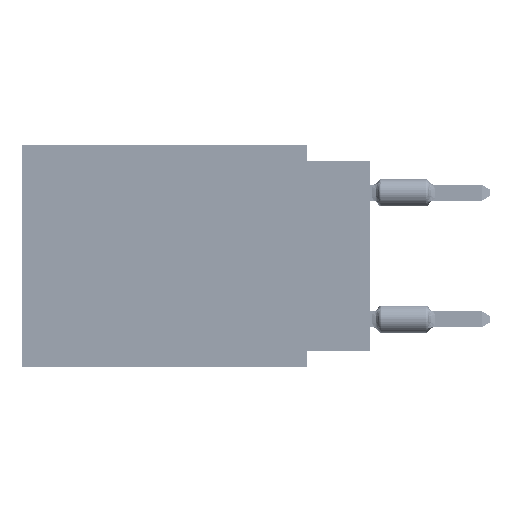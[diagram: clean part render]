
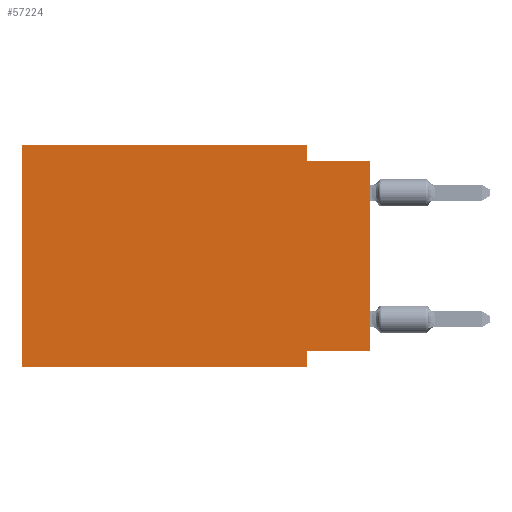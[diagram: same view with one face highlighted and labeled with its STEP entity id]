
A CAD part, left-side view. The second image highlights one B-rep face of the part: STEP entity #57224.
In plain terms, the highlighted planar face has unit normal (-1, 0, 0).
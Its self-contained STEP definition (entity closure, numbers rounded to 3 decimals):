
#6 = CARTESIAN_POINT ( 'NONE',  ( 0., 0., -8.255 ) ) ;
#1373 = CARTESIAN_POINT ( 'NONE',  ( 0., 13.97, -8.89 ) ) ;
#1669 = DIRECTION ( 'NONE',  ( 0., -1., 0. ) ) ;
#2121 = CARTESIAN_POINT ( 'NONE',  ( 0., 13.97, 0. ) ) ;
#2749 = VECTOR ( 'NONE', #61164, 1000. ) ;
#2925 = VERTEX_POINT ( 'NONE', #60338 ) ;
#3912 = VECTOR ( 'NONE', #45170, 1000. ) ;
#4135 = VERTEX_POINT ( 'NONE', #33425 ) ;
#4671 = ORIENTED_EDGE ( 'NONE', *, *, #45342, .F. ) ;
#5426 = VECTOR ( 'NONE', #49405, 1000. ) ;
#6411 = VECTOR ( 'NONE', #42170, 1000. ) ;
#7869 = VERTEX_POINT ( 'NONE', #43245 ) ;
#8505 = VECTOR ( 'NONE', #1669, 1000. ) ;
#12434 = EDGE_LOOP ( 'NONE', ( #36051, #48509, #4671, #23548, #65354, #19187, #33474, #23314 ) ) ;
#13574 = DIRECTION ( 'NONE',  ( 1., 0., 0. ) ) ;
#13712 = LINE ( 'NONE', #67675, #30458 ) ;
#14795 = VERTEX_POINT ( 'NONE', #1373 ) ;
#16753 = VERTEX_POINT ( 'NONE', #24791 ) ;
#18209 = PLANE ( 'NONE',  #68931 ) ;
#19187 = ORIENTED_EDGE ( 'NONE', *, *, #57685, .T. ) ;
#23314 = ORIENTED_EDGE ( 'NONE', *, *, #55597, .F. ) ;
#23548 = ORIENTED_EDGE ( 'NONE', *, *, #30629, .F. ) ;
#23978 = LINE ( 'NONE', #46835, #34636 ) ;
#24791 = CARTESIAN_POINT ( 'NONE',  ( 0., 2.54, -8.255 ) ) ;
#28027 = DIRECTION ( 'NONE',  ( 0., -1., 0. ) ) ;
#29636 = FACE_OUTER_BOUND ( 'NONE', #12434, .T. ) ;
#30458 = VECTOR ( 'NONE', #46916, 1000. ) ;
#30629 = EDGE_CURVE ( 'NONE', #2925, #41798, #59669, .T. ) ;
#33425 = CARTESIAN_POINT ( 'NONE',  ( 0., 2.54, -8.89 ) ) ;
#33474 = ORIENTED_EDGE ( 'NONE', *, *, #55170, .F. ) ;
#34028 = CARTESIAN_POINT ( 'NONE',  ( 0., 0., 0. ) ) ;
#34437 = LINE ( 'NONE', #40511, #3912 ) ;
#34636 = VECTOR ( 'NONE', #28027, 1000. ) ;
#36051 = ORIENTED_EDGE ( 'NONE', *, *, #60522, .T. ) ;
#38106 = VECTOR ( 'NONE', #42697, 1000. ) ;
#38647 = LINE ( 'NONE', #39332, #2749 ) ;
#39332 = CARTESIAN_POINT ( 'NONE',  ( 0., 0., -8.255 ) ) ;
#40489 = CARTESIAN_POINT ( 'NONE',  ( 0., 2.54, -0.635 ) ) ;
#40511 = CARTESIAN_POINT ( 'NONE',  ( 0., 13.97, 0. ) ) ;
#41798 = VERTEX_POINT ( 'NONE', #46717 ) ;
#42170 = DIRECTION ( 'NONE',  ( 0., -1., 0. ) ) ;
#42697 = DIRECTION ( 'NONE',  ( 0., 0., -1. ) ) ;
#43245 = CARTESIAN_POINT ( 'NONE',  ( 0., 0., -0.635 ) ) ;
#45170 = DIRECTION ( 'NONE',  ( 0., 0., 1. ) ) ;
#45342 = EDGE_CURVE ( 'NONE', #41798, #52686, #13712, .T. ) ;
#46717 = CARTESIAN_POINT ( 'NONE',  ( 0., 2.54, 0. ) ) ;
#46835 = CARTESIAN_POINT ( 'NONE',  ( 0., 0., -0.635 ) ) ;
#46916 = DIRECTION ( 'NONE',  ( 0., 0., -1. ) ) ;
#48509 = ORIENTED_EDGE ( 'NONE', *, *, #54257, .F. ) ;
#49405 = DIRECTION ( 'NONE',  ( 0., 0., 1. ) ) ;
#50657 = CARTESIAN_POINT ( 'NONE',  ( 0., 13.97, -8.89 ) ) ;
#52686 = VERTEX_POINT ( 'NONE', #40489 ) ;
#52897 = CARTESIAN_POINT ( 'NONE',  ( 0., 13.97, 0. ) ) ;
#53462 = CARTESIAN_POINT ( 'NONE',  ( 0., 2.54, -8.89 ) ) ;
#54257 = EDGE_CURVE ( 'NONE', #52686, #7869, #23978, .T. ) ;
#54431 = LINE ( 'NONE', #34028, #5426 ) ;
#55170 = EDGE_CURVE ( 'NONE', #16753, #4135, #68488, .T. ) ;
#55456 = EDGE_CURVE ( 'NONE', #14795, #2925, #34437, .T. ) ;
#55597 = EDGE_CURVE ( 'NONE', #55898, #16753, #38647, .T. ) ;
#55898 = VERTEX_POINT ( 'NONE', #6 ) ;
#57224 = ADVANCED_FACE ( 'NONE', ( #29636 ), #18209, .F. ) ;
#57685 = EDGE_CURVE ( 'NONE', #14795, #4135, #63136, .T. ) ;
#59669 = LINE ( 'NONE', #52897, #6411 ) ;
#60338 = CARTESIAN_POINT ( 'NONE',  ( 0., 13.97, 0. ) ) ;
#60522 = EDGE_CURVE ( 'NONE', #55898, #7869, #54431, .T. ) ;
#61164 = DIRECTION ( 'NONE',  ( 0., 1., 0. ) ) ;
#62885 = DIRECTION ( 'NONE',  ( 0., 0., -1. ) ) ;
#63136 = LINE ( 'NONE', #50657, #8505 ) ;
#65354 = ORIENTED_EDGE ( 'NONE', *, *, #55456, .F. ) ;
#67675 = CARTESIAN_POINT ( 'NONE',  ( 0., 2.54, 0. ) ) ;
#68488 = LINE ( 'NONE', #53462, #38106 ) ;
#68931 = AXIS2_PLACEMENT_3D ( 'NONE', #2121, #13574, #62885 ) ;
